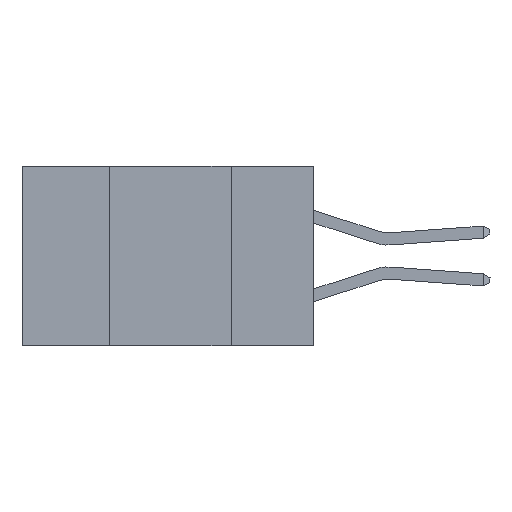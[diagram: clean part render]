
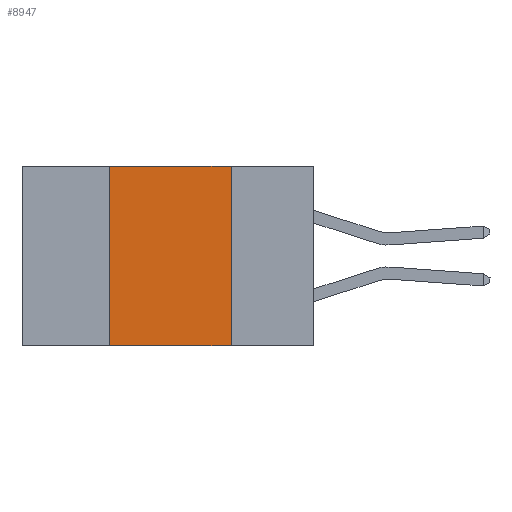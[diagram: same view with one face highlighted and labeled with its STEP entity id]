
A CAD part, left-side view. The second image highlights one B-rep face of the part: STEP entity #8947.
In plain terms, the highlighted planar face has unit normal (-1, 0, 0).
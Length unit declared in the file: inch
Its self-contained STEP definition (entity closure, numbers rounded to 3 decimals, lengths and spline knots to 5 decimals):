
#304 = ORIENTED_EDGE ( 'NONE', *, *, #5757, .F. ) ;
#487 = AXIS2_PLACEMENT_3D ( 'NONE', #1687, #8761, #623 ) ;
#499 = EDGE_CURVE ( 'NONE', #8331, #14551, #7019, .T. ) ;
#623 = DIRECTION ( 'NONE',  ( 0., 0., -1. ) ) ;
#841 = CARTESIAN_POINT ( 'NONE',  ( 0., 0.6, 0. ) ) ;
#1125 = CARTESIAN_POINT ( 'NONE',  ( 0., 0.42, -0.37 ) ) ;
#1544 = VECTOR ( 'NONE', #2126, 39.37008 ) ;
#1687 = CARTESIAN_POINT ( 'NONE',  ( 0., 0.6, 0. ) ) ;
#1813 = ORIENTED_EDGE ( 'NONE', *, *, #7646, .F. ) ;
#2126 = DIRECTION ( 'NONE',  ( 0., 0., -1. ) ) ;
#2485 = CARTESIAN_POINT ( 'NONE',  ( 0., 0.17, -0.37 ) ) ;
#4084 = ORIENTED_EDGE ( 'NONE', *, *, #4332, .T. ) ;
#4332 = EDGE_CURVE ( 'NONE', #7962, #14551, #13529, .T. ) ;
#4888 = CARTESIAN_POINT ( 'NONE',  ( 0., 0.6, -0.37 ) ) ;
#5359 = LINE ( 'NONE', #841, #15917 ) ;
#5757 = EDGE_CURVE ( 'NONE', #16816, #8331, #5359, .T. ) ;
#6054 = EDGE_LOOP ( 'NONE', ( #18004, #304, #1813, #4084 ) ) ;
#6636 = CARTESIAN_POINT ( 'NONE',  ( 0., 0.17, 0. ) ) ;
#7019 = LINE ( 'NONE', #13540, #1544 ) ;
#7411 = VECTOR ( 'NONE', #14778, 39.37008 ) ;
#7646 = EDGE_CURVE ( 'NONE', #7962, #16816, #15775, .T. ) ;
#7962 = VERTEX_POINT ( 'NONE', #1125 ) ;
#8331 = VERTEX_POINT ( 'NONE', #6636 ) ;
#8761 = DIRECTION ( 'NONE',  ( 1., 0., 0. ) ) ;
#8947 = ADVANCED_FACE ( 'NONE', ( #10295 ), #9972, .F. ) ;
#9830 = VECTOR ( 'NONE', #12379, 39.37008 ) ;
#9972 = PLANE ( 'NONE',  #487 ) ;
#10295 = FACE_OUTER_BOUND ( 'NONE', #6054, .T. ) ;
#10771 = CARTESIAN_POINT ( 'NONE',  ( 0., 0.42, 0. ) ) ;
#12379 = DIRECTION ( 'NONE',  ( 0., 0., 1. ) ) ;
#12426 = CARTESIAN_POINT ( 'NONE',  ( 0., 0.42, 0. ) ) ;
#13529 = LINE ( 'NONE', #4888, #7411 ) ;
#13540 = CARTESIAN_POINT ( 'NONE',  ( 0., 0.17, 0. ) ) ;
#14551 = VERTEX_POINT ( 'NONE', #2485 ) ;
#14723 = DIRECTION ( 'NONE',  ( 0., -1., 0. ) ) ;
#14778 = DIRECTION ( 'NONE',  ( 0., -1., 0. ) ) ;
#15775 = LINE ( 'NONE', #10771, #9830 ) ;
#15917 = VECTOR ( 'NONE', #14723, 39.37008 ) ;
#16816 = VERTEX_POINT ( 'NONE', #12426 ) ;
#18004 = ORIENTED_EDGE ( 'NONE', *, *, #499, .F. ) ;
